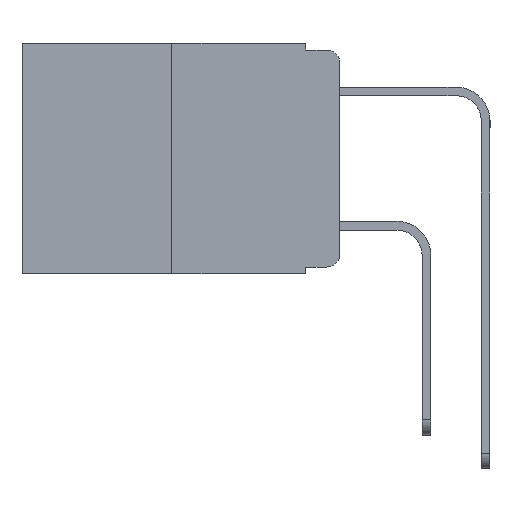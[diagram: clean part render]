
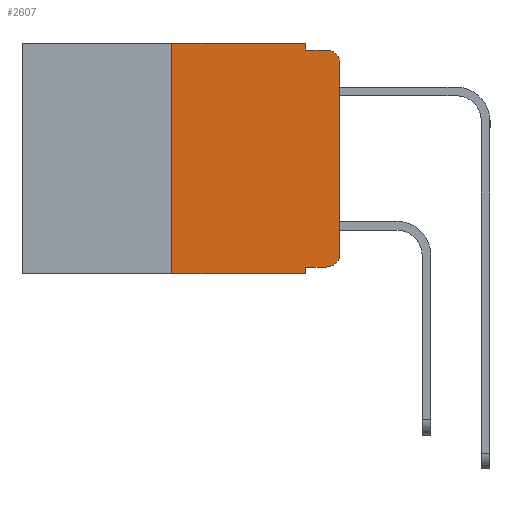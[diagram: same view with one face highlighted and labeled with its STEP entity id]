
A CAD part, left-side view. The second image highlights one B-rep face of the part: STEP entity #2607.
In plain terms, the highlighted planar face has unit normal (-1, 0, 0).
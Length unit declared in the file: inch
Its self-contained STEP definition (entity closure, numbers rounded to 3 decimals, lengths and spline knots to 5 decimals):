
#43 = ORIENTED_EDGE ( 'NONE', *, *, #13007, .T. ) ;
#316 = CARTESIAN_POINT ( 'NONE',  ( 0., 0.051, -0.01 ) ) ;
#889 = VERTEX_POINT ( 'NONE', #9596 ) ;
#944 = VECTOR ( 'NONE', #10957, 39.37008 ) ;
#971 = EDGE_LOOP ( 'NONE', ( #8961, #2980, #15241, #19962, #995, #1596, #11340, #3533, #43, #10411 ) ) ;
#995 = ORIENTED_EDGE ( 'NONE', *, *, #9187, .F. ) ;
#1596 = ORIENTED_EDGE ( 'NONE', *, *, #7521, .F. ) ;
#2607 = ADVANCED_FACE ( 'NONE', ( #6853 ), #12505, .F. ) ;
#2980 = ORIENTED_EDGE ( 'NONE', *, *, #7459, .T. ) ;
#3185 = LINE ( 'NONE', #15691, #10598 ) ;
#3433 = AXIS2_PLACEMENT_3D ( 'NONE', #17998, #9178, #19410 ) ;
#3533 = ORIENTED_EDGE ( 'NONE', *, *, #4870, .F. ) ;
#4074 = DIRECTION ( 'NONE',  ( 0., 0., -1. ) ) ;
#4213 = VERTEX_POINT ( 'NONE', #6649 ) ;
#4855 = DIRECTION ( 'NONE',  ( -1., 0., 0. ) ) ;
#4870 = EDGE_CURVE ( 'NONE', #889, #5421, #3185, .T. ) ;
#5061 = DIRECTION ( 'NONE',  ( 0., 0., -1. ) ) ;
#5070 = CARTESIAN_POINT ( 'NONE',  ( 0., 0.051, -0.01 ) ) ;
#5421 = VERTEX_POINT ( 'NONE', #6926 ) ;
#5438 = VECTOR ( 'NONE', #5554, 39.37008 ) ;
#5490 = LINE ( 'NONE', #6483, #17022 ) ;
#5554 = DIRECTION ( 'NONE',  ( 0., -1., 0. ) ) ;
#5850 = VERTEX_POINT ( 'NONE', #16123 ) ;
#5890 = CARTESIAN_POINT ( 'NONE',  ( 0., 0., -0.313 ) ) ;
#5952 = LINE ( 'NONE', #316, #5438 ) ;
#6413 = EDGE_CURVE ( 'NONE', #10743, #20093, #17552, .T. ) ;
#6483 = CARTESIAN_POINT ( 'NONE',  ( 0., 0.473, -0.343 ) ) ;
#6649 = CARTESIAN_POINT ( 'NONE',  ( 0., 0.25, 0. ) ) ;
#6853 = FACE_OUTER_BOUND ( 'NONE', #971, .T. ) ;
#6926 = CARTESIAN_POINT ( 'NONE',  ( 0., 0.051, -0.343 ) ) ;
#7459 = EDGE_CURVE ( 'NONE', #9942, #15125, #14561, .T. ) ;
#7521 = EDGE_CURVE ( 'NONE', #9321, #4213, #10624, .T. ) ;
#7559 = VERTEX_POINT ( 'NONE', #5070 ) ;
#7893 = VECTOR ( 'NONE', #19152, 39.37008 ) ;
#7935 = CARTESIAN_POINT ( 'NONE',  ( 0., 0.051, 0. ) ) ;
#8009 = DIRECTION ( 'NONE',  ( 0., -1., 0. ) ) ;
#8961 = ORIENTED_EDGE ( 'NONE', *, *, #14685, .T. ) ;
#9178 = DIRECTION ( 'NONE',  ( -1., 0., 0. ) ) ;
#9187 = EDGE_CURVE ( 'NONE', #4213, #5850, #15873, .T. ) ;
#9287 = CARTESIAN_POINT ( 'NONE',  ( 0., 0.25, -0.343 ) ) ;
#9321 = VERTEX_POINT ( 'NONE', #9287 ) ;
#9458 = DIRECTION ( 'NONE',  ( 0., -1., 0. ) ) ;
#9596 = CARTESIAN_POINT ( 'NONE',  ( 0., 0.051, -0.333 ) ) ;
#9664 = LINE ( 'NONE', #7935, #944 ) ;
#9671 = CARTESIAN_POINT ( 'NONE',  ( 0., 0., 0. ) ) ;
#9776 = EDGE_CURVE ( 'NONE', #7559, #15125, #5952, .T. ) ;
#9942 = VERTEX_POINT ( 'NONE', #12253 ) ;
#10200 = DIRECTION ( 'NONE',  ( 1., 0., 0. ) ) ;
#10411 = ORIENTED_EDGE ( 'NONE', *, *, #6413, .T. ) ;
#10598 = VECTOR ( 'NONE', #5061, 39.37008 ) ;
#10624 = LINE ( 'NONE', #18469, #17047 ) ;
#10743 = VERTEX_POINT ( 'NONE', #16773 ) ;
#10858 = CARTESIAN_POINT ( 'NONE',  ( 0., 0.473, 0. ) ) ;
#10957 = DIRECTION ( 'NONE',  ( 0., 0., -1. ) ) ;
#11106 = AXIS2_PLACEMENT_3D ( 'NONE', #10858, #10200, #4074 ) ;
#11110 = LINE ( 'NONE', #18259, #11571 ) ;
#11340 = ORIENTED_EDGE ( 'NONE', *, *, #14659, .T. ) ;
#11410 = AXIS2_PLACEMENT_3D ( 'NONE', #14026, #4855, #15499 ) ;
#11571 = VECTOR ( 'NONE', #9458, 39.37008 ) ;
#12253 = CARTESIAN_POINT ( 'NONE',  ( 0., 0., -0.03 ) ) ;
#12505 = PLANE ( 'NONE',  #11106 ) ;
#12663 = LINE ( 'NONE', #9671, #19920 ) ;
#13007 = EDGE_CURVE ( 'NONE', #889, #10743, #11110, .T. ) ;
#14026 = CARTESIAN_POINT ( 'NONE',  ( 0., 0.02, -0.03 ) ) ;
#14561 = CIRCLE ( 'NONE', #11410, 0.02 ) ;
#14635 = EDGE_CURVE ( 'NONE', #5850, #7559, #9664, .T. ) ;
#14659 = EDGE_CURVE ( 'NONE', #9321, #5421, #5490, .T. ) ;
#14685 = EDGE_CURVE ( 'NONE', #20093, #9942, #12663, .T. ) ;
#15125 = VERTEX_POINT ( 'NONE', #16245 ) ;
#15241 = ORIENTED_EDGE ( 'NONE', *, *, #9776, .F. ) ;
#15499 = DIRECTION ( 'NONE',  ( 0., 0., -1. ) ) ;
#15691 = CARTESIAN_POINT ( 'NONE',  ( 0., 0.051, 0. ) ) ;
#15873 = LINE ( 'NONE', #17725, #7893 ) ;
#16123 = CARTESIAN_POINT ( 'NONE',  ( 0., 0.051, 0. ) ) ;
#16245 = CARTESIAN_POINT ( 'NONE',  ( 0., 0.02, -0.01 ) ) ;
#16773 = CARTESIAN_POINT ( 'NONE',  ( 0., 0.02, -0.333 ) ) ;
#17022 = VECTOR ( 'NONE', #8009, 39.37008 ) ;
#17047 = VECTOR ( 'NONE', #19877, 39.37008 ) ;
#17552 = CIRCLE ( 'NONE', #3433, 0.02 ) ;
#17725 = CARTESIAN_POINT ( 'NONE',  ( 0., 0.473, 0. ) ) ;
#17998 = CARTESIAN_POINT ( 'NONE',  ( 0., 0.02, -0.313 ) ) ;
#18259 = CARTESIAN_POINT ( 'NONE',  ( 0., 0.051, -0.333 ) ) ;
#18469 = CARTESIAN_POINT ( 'NONE',  ( 0., 0.25, 0. ) ) ;
#19152 = DIRECTION ( 'NONE',  ( 0., -1., 0. ) ) ;
#19410 = DIRECTION ( 'NONE',  ( 0., 0., -1. ) ) ;
#19862 = DIRECTION ( 'NONE',  ( 0., 0., 1. ) ) ;
#19877 = DIRECTION ( 'NONE',  ( 0., 0., 1. ) ) ;
#19920 = VECTOR ( 'NONE', #19862, 39.37008 ) ;
#19962 = ORIENTED_EDGE ( 'NONE', *, *, #14635, .F. ) ;
#20093 = VERTEX_POINT ( 'NONE', #5890 ) ;
